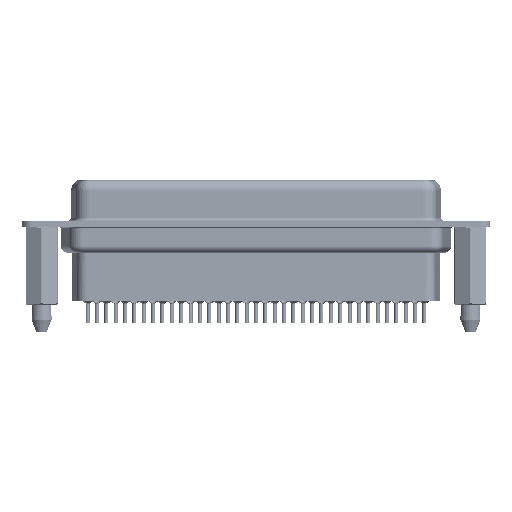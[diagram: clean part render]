
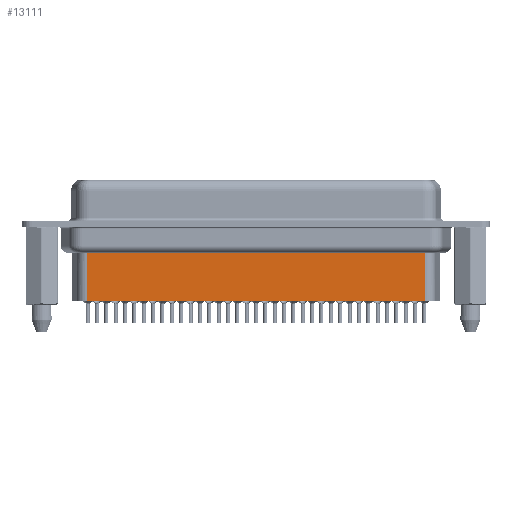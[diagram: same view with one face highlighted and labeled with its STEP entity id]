
A CAD part, front view. The second image highlights one B-rep face of the part: STEP entity #13111.
In plain terms, the highlighted planar face has unit normal (0, -1, 0).
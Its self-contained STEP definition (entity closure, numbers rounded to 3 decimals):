
#24 = ORIENTED_EDGE ( 'NONE', *, *, #7116, .T. ) ;
#624 = DIRECTION ( 'NONE',  ( -1., 0., 0. ) ) ;
#1128 = VERTEX_POINT ( 'NONE', #17094 ) ;
#3376 = EDGE_LOOP ( 'NONE', ( #20404, #30851, #24, #26546 ) ) ;
#4009 = DIRECTION ( 'NONE',  ( 0., -1., 0. ) ) ;
#4516 = FACE_OUTER_BOUND ( 'NONE', #3376, .T. ) ;
#5962 = CARTESIAN_POINT ( 'NONE',  ( 6.706, -3.5, -11.45 ) ) ;
#6435 = LINE ( 'NONE', #10239, #20120 ) ;
#7116 = EDGE_CURVE ( 'NONE', #19485, #1128, #6435, .T. ) ;
#7460 = DIRECTION ( 'NONE',  ( 0., 0., -1. ) ) ;
#8819 = EDGE_CURVE ( 'NONE', #30158, #19485, #15343, .T. ) ;
#8869 = CARTESIAN_POINT ( 'NONE',  ( 56.794, -3.5, -4.097 ) ) ;
#8881 = LINE ( 'NONE', #25930, #22546 ) ;
#10239 = CARTESIAN_POINT ( 'NONE',  ( 6.706, -3.5, -3.1 ) ) ;
#12508 = DIRECTION ( 'NONE',  ( 0., 0., -1. ) ) ;
#12598 = CARTESIAN_POINT ( 'NONE',  ( 56.794, -3.5, -11.45 ) ) ;
#13111 = ADVANCED_FACE ( 'NONE', ( #4516 ), #20319, .T. ) ;
#15343 = LINE ( 'NONE', #33871, #29485 ) ;
#15355 = DIRECTION ( 'NONE',  ( -1., 0., 0. ) ) ;
#17094 = CARTESIAN_POINT ( 'NONE',  ( 6.706, -3.5, -11.45 ) ) ;
#19100 = VECTOR ( 'NONE', #624, 1000. ) ;
#19485 = VERTEX_POINT ( 'NONE', #33740 ) ;
#20120 = VECTOR ( 'NONE', #7460, 1000. ) ;
#20319 = PLANE ( 'NONE',  #32269 ) ;
#20404 = ORIENTED_EDGE ( 'NONE', *, *, #27368, .F. ) ;
#21406 = VERTEX_POINT ( 'NONE', #12598 ) ;
#22546 = VECTOR ( 'NONE', #12508, 1000. ) ;
#23002 = DIRECTION ( 'NONE',  ( 1., 0., 0. ) ) ;
#25930 = CARTESIAN_POINT ( 'NONE',  ( 56.794, -3.5, -3.1 ) ) ;
#26546 = ORIENTED_EDGE ( 'NONE', *, *, #28682, .F. ) ;
#27368 = EDGE_CURVE ( 'NONE', #30158, #21406, #8881, .T. ) ;
#28682 = EDGE_CURVE ( 'NONE', #21406, #1128, #32321, .T. ) ;
#29485 = VECTOR ( 'NONE', #15355, 1000. ) ;
#30158 = VERTEX_POINT ( 'NONE', #8869 ) ;
#30644 = CARTESIAN_POINT ( 'NONE',  ( 6.706, -3.5, -3.1 ) ) ;
#30851 = ORIENTED_EDGE ( 'NONE', *, *, #8819, .T. ) ;
#32269 = AXIS2_PLACEMENT_3D ( 'NONE', #30644, #4009, #23002 ) ;
#32321 = LINE ( 'NONE', #5962, #19100 ) ;
#33740 = CARTESIAN_POINT ( 'NONE',  ( 6.706, -3.5, -4.097 ) ) ;
#33871 = CARTESIAN_POINT ( 'NONE',  ( 6.459, -3.5, -4.097 ) ) ;
